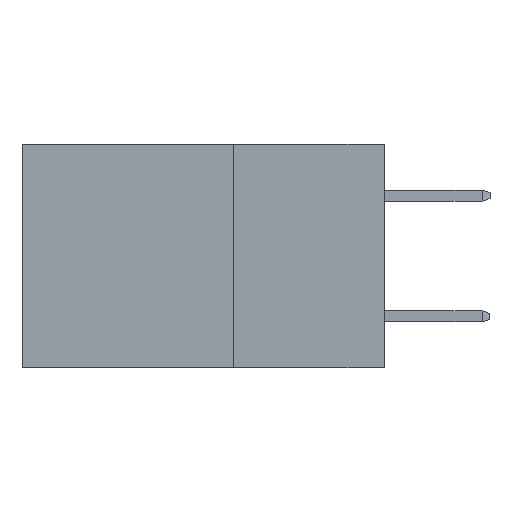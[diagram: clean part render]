
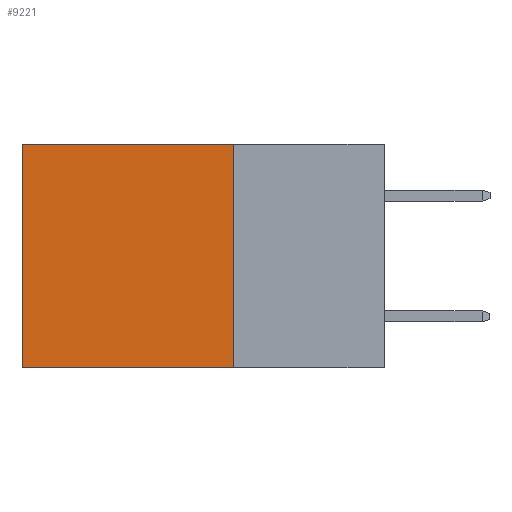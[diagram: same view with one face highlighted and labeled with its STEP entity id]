
A CAD part, left-side view. The second image highlights one B-rep face of the part: STEP entity #9221.
In plain terms, the highlighted planar face has unit normal (-1, 0, 0).
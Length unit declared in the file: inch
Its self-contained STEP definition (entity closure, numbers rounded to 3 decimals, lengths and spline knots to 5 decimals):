
#113 = FACE_OUTER_BOUND ( 'NONE', #5698, .T. ) ;
#550 = DIRECTION ( 'NONE',  ( 1., 0., 0. ) ) ;
#2026 = ORIENTED_EDGE ( 'NONE', *, *, #4222, .T. ) ;
#2181 = ORIENTED_EDGE ( 'NONE', *, *, #8229, .F. ) ;
#2394 = ORIENTED_EDGE ( 'NONE', *, *, #6164, .F. ) ;
#2462 = ORIENTED_EDGE ( 'NONE', *, *, #6055, .T. ) ;
#3430 = VECTOR ( 'NONE', #11603, 39.37008 ) ;
#3716 = CARTESIAN_POINT ( 'NONE',  ( 0.298, 0.25, 0. ) ) ;
#4222 = EDGE_CURVE ( 'NONE', #10209, #13156, #6167, .T. ) ;
#4263 = VERTEX_POINT ( 'NONE', #5376 ) ;
#4604 = LINE ( 'NONE', #9163, #12048 ) ;
#4618 = CARTESIAN_POINT ( 'NONE',  ( 0.298, 0.25, 0. ) ) ;
#5376 = CARTESIAN_POINT ( 'NONE',  ( 0.298, 0.25, 0. ) ) ;
#5449 = VERTEX_POINT ( 'NONE', #8904 ) ;
#5645 = CARTESIAN_POINT ( 'NONE',  ( 0.298, 0.6, 0. ) ) ;
#5698 = EDGE_LOOP ( 'NONE', ( #2026, #2181, #2394, #2462 ) ) ;
#5741 = AXIS2_PLACEMENT_3D ( 'NONE', #9706, #550, #7715 ) ;
#6055 = EDGE_CURVE ( 'NONE', #4263, #10209, #11171, .T. ) ;
#6164 = EDGE_CURVE ( 'NONE', #4263, #5449, #10257, .T. ) ;
#6167 = LINE ( 'NONE', #5645, #3430 ) ;
#6626 = CARTESIAN_POINT ( 'NONE',  ( 0.298, 0.6, -0.37 ) ) ;
#6678 = PLANE ( 'NONE',  #5741 ) ;
#7168 = CARTESIAN_POINT ( 'NONE',  ( 0.298, 0.6, 0. ) ) ;
#7715 = DIRECTION ( 'NONE',  ( 0., 0., -1. ) ) ;
#8229 = EDGE_CURVE ( 'NONE', #5449, #13156, #4604, .T. ) ;
#8904 = CARTESIAN_POINT ( 'NONE',  ( 0.298, 0.25, -0.37 ) ) ;
#9163 = CARTESIAN_POINT ( 'NONE',  ( 0.298, 0.25, -0.37 ) ) ;
#9221 = ADVANCED_FACE ( 'NONE', ( #113 ), #6678, .F. ) ;
#9599 = VECTOR ( 'NONE', #11794, 39.37008 ) ;
#9706 = CARTESIAN_POINT ( 'NONE',  ( 0.298, 0.25, 0. ) ) ;
#10197 = DIRECTION ( 'NONE',  ( 0., 1., 0. ) ) ;
#10209 = VERTEX_POINT ( 'NONE', #7168 ) ;
#10257 = LINE ( 'NONE', #3716, #9599 ) ;
#10872 = VECTOR ( 'NONE', #12732, 39.37008 ) ;
#11171 = LINE ( 'NONE', #4618, #10872 ) ;
#11603 = DIRECTION ( 'NONE',  ( 0., 0., -1. ) ) ;
#11794 = DIRECTION ( 'NONE',  ( 0., 0., -1. ) ) ;
#12048 = VECTOR ( 'NONE', #10197, 39.37008 ) ;
#12732 = DIRECTION ( 'NONE',  ( 0., 1., 0. ) ) ;
#13156 = VERTEX_POINT ( 'NONE', #6626 ) ;
